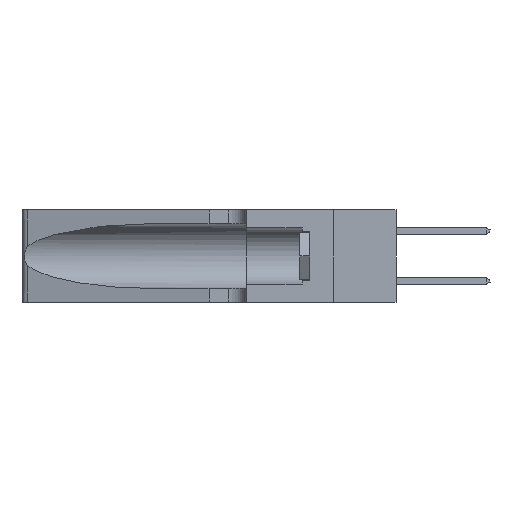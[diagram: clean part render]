
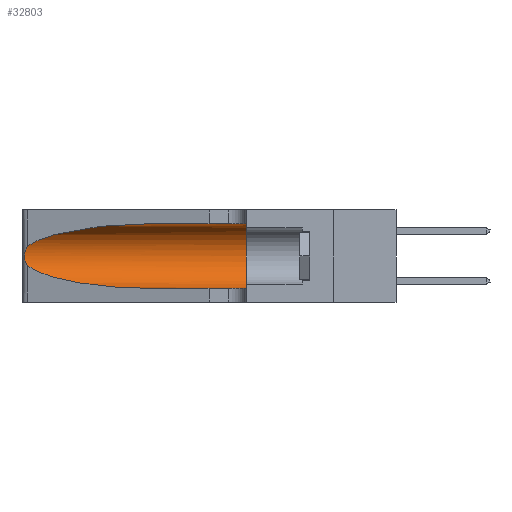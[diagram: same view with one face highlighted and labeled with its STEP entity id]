
A CAD part, left-side view. The second image highlights one B-rep face of the part: STEP entity #32803.
In plain terms, the highlighted cylindrical face has radius 3.308 mm (diameter 6.617 mm), a partial arc.
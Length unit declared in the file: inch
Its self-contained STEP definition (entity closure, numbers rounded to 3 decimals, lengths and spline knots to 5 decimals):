
#409 = VERTEX_POINT ( 'NONE', #32233 ) ;
#2786 = CARTESIAN_POINT ( 'NONE',  ( 0.26017, 1.23833, 0.17102 ) ) ;
#2938 = CARTESIAN_POINT ( 'NONE',  ( 0.25854, 1.2359, 0.20912 ) ) ;
#4188 = AXIS2_PLACEMENT_3D ( 'NONE', #8085, #33717, #25704 ) ;
#4823 = EDGE_CURVE ( 'NONE', #28639, #14928, #31221, .T. ) ;
#6222 = DIRECTION ( 'NONE',  ( 0., -1., 0. ) ) ;
#6497 = ORIENTED_EDGE ( 'NONE', *, *, #22093, .F. ) ;
#6496 = CARTESIAN_POINT ( 'NONE',  ( 0.25789, 1.23486, 0.15765 ) ) ;
#8085 = CARTESIAN_POINT ( 'NONE',  ( 0.1305, 0.35, 0.185 ) ) ;
#8972 = ORIENTED_EDGE ( 'NONE', *, *, #34761, .T. ) ;
#9079 = CARTESIAN_POINT ( 'NONE',  ( 0.1305, 0.35, 0.31525 ) ) ;
#9128 = LINE ( 'NONE', #35742, #40098 ) ;
#10002 = CARTESIAN_POINT ( 'NONE',  ( 0.25487, 1.22718, 0.14631 ) ) ;
#11672 = CARTESIAN_POINT ( 'NONE',  ( 0.18966, 0.96281, 0.31525 ) ) ;
#11804 = DIRECTION ( 'NONE',  ( 0., -1., 0. ) ) ;
#11962 = CARTESIAN_POINT ( 'NONE',  ( 0.1305, 1.61858, 0.185 ) ) ;
#14061 = CARTESIAN_POINT ( 'NONE',  ( 0.26018, 1.23835, 0.19895 ) ) ;
#14373 = CARTESIAN_POINT ( 'NONE',  ( 0.26075, 1.23896, 0.19203 ) ) ;
#14928 = VERTEX_POINT ( 'NONE', #27453 ) ;
#16076 = EDGE_LOOP ( 'NONE', ( #20208, #30236, #8972, #41816, #6497, #32143 ) ) ;
#16143 = VERTEX_POINT ( 'NONE', #9079 ) ;
#17191 = B_SPLINE_CURVE_WITH_KNOTS ( 'NONE', 3,
 ( #43513, #24772, #29067, #46709, #2938, #14061, #14373, #25227, #2786, #21719, #6496, #39848, #32140, #28915 ),
 .UNSPECIFIED., .F., .F.,
 ( 4, 2, 2, 2, 2, 2, 4 ),
 ( 0., 0.00027, 0.00053, 0.00107, 0.0016, 0.00187, 0.00214 ),
 .UNSPECIFIED. ) ;
#17555 = CARTESIAN_POINT ( 'NONE',  ( 0.18966, 0.96281, 0.05475 ) ) ;
#17965 = EDGE_CURVE ( 'NONE', #409, #37661, #17191, .T. ) ;
#18624 =( BOUNDED_CURVE ( )  B_SPLINE_CURVE ( 3, ( #10002, #20283, #17555, #21398 ),
 .UNSPECIFIED., .F., .T. ) 
 B_SPLINE_CURVE_WITH_KNOTS ( ( 4, 4 ),
 ( 3.44316, 4.71239 ),
 .UNSPECIFIED. ) 
 CURVE ( )  GEOMETRIC_REPRESENTATION_ITEM ( )  RATIONAL_B_SPLINE_CURVE ( ( 1., 0.87, 0.87, 1. ) ) 
 REPRESENTATION_ITEM ( '' )  );
#19201 = CARTESIAN_POINT ( 'NONE',  ( 0.1305, 0.72297, 0.31525 ) ) ;
#19380 = EDGE_CURVE ( 'NONE', #37671, #409, #31523, .T. ) ;
#20208 = ORIENTED_EDGE ( 'NONE', *, *, #19380, .T. ) ;
#20212 = CARTESIAN_POINT ( 'NONE',  ( 0.1305, 0.72297, 0.31525 ) ) ;
#20283 = CARTESIAN_POINT ( 'NONE',  ( 0.2373, 1.15595, 0.08982 ) ) ;
#21169 = EDGE_CURVE ( 'NONE', #37671, #16143, #9128, .T. ) ;
#21398 = CARTESIAN_POINT ( 'NONE',  ( 0.1305, 0.72297, 0.05475 ) ) ;
#21719 = CARTESIAN_POINT ( 'NONE',  ( 0.25856, 1.23593, 0.16098 ) ) ;
#22093 = EDGE_CURVE ( 'NONE', #16143, #14928, #23360, .T. ) ;
#23360 = CIRCLE ( 'NONE', #4188, 0.13025 ) ;
#23750 = CARTESIAN_POINT ( 'NONE',  ( 0.25487, 1.22718, 0.14631 ) ) ;
#24772 = CARTESIAN_POINT ( 'NONE',  ( 0.25555, 1.22994, 0.2215 ) ) ;
#25227 = CARTESIAN_POINT ( 'NONE',  ( 0.26075, 1.23896, 0.178 ) ) ;
#25704 = DIRECTION ( 'NONE',  ( 0., 0., 1. ) ) ;
#26779 = DIRECTION ( 'NONE',  ( 0., -1., 0. ) ) ;
#27453 = CARTESIAN_POINT ( 'NONE',  ( 0.1305, 0.35, 0.05475 ) ) ;
#28639 = VERTEX_POINT ( 'NONE', #34189 ) ;
#28915 = CARTESIAN_POINT ( 'NONE',  ( 0.25487, 1.22718, 0.14631 ) ) ;
#29067 = CARTESIAN_POINT ( 'NONE',  ( 0.25639, 1.23184, 0.21858 ) ) ;
#29583 = CARTESIAN_POINT ( 'NONE',  ( 0.2373, 1.15595, 0.28018 ) ) ;
#30045 = VECTOR ( 'NONE', #26779, 39.37008 ) ;
#30065 = CARTESIAN_POINT ( 'NONE',  ( 0.25487, 1.22718, 0.22369 ) ) ;
#30236 = ORIENTED_EDGE ( 'NONE', *, *, #17965, .T. ) ;
#31221 = LINE ( 'NONE', #41539, #30045 ) ;
#31523 =( BOUNDED_CURVE ( )  B_SPLINE_CURVE ( 3, ( #19201, #11672, #29583, #30065 ),
 .UNSPECIFIED., .F., .F. ) 
 B_SPLINE_CURVE_WITH_KNOTS ( ( 4, 4 ),
 ( 1.5708, 2.84003 ),
 .UNSPECIFIED. ) 
 CURVE ( )  GEOMETRIC_REPRESENTATION_ITEM ( )  RATIONAL_B_SPLINE_CURVE ( ( 1., 0.87, 0.87, 1. ) ) 
 REPRESENTATION_ITEM ( '' )  );
#32140 = CARTESIAN_POINT ( 'NONE',  ( 0.25555, 1.22993, 0.14849 ) ) ;
#32143 = ORIENTED_EDGE ( 'NONE', *, *, #21169, .F. ) ;
#32233 = CARTESIAN_POINT ( 'NONE',  ( 0.25487, 1.22718, 0.22369 ) ) ;
#32803 = ADVANCED_FACE ( 'NONE', ( #33558 ), #43322, .F. ) ;
#33558 = FACE_OUTER_BOUND ( 'NONE', #16076, .T. ) ;
#33717 = DIRECTION ( 'NONE',  ( 0., 1., 0. ) ) ;
#34189 = CARTESIAN_POINT ( 'NONE',  ( 0.1305, 0.72297, 0.05475 ) ) ;
#34761 = EDGE_CURVE ( 'NONE', #37661, #28639, #18624, .T. ) ;
#35742 = CARTESIAN_POINT ( 'NONE',  ( 0.1305, 1.61858, 0.31525 ) ) ;
#37469 = DIRECTION ( 'NONE',  ( 0., 0., -1. ) ) ;
#37661 = VERTEX_POINT ( 'NONE', #23750 ) ;
#37671 = VERTEX_POINT ( 'NONE', #20212 ) ;
#39828 = AXIS2_PLACEMENT_3D ( 'NONE', #11962, #11804, #37469 ) ;
#39848 = CARTESIAN_POINT ( 'NONE',  ( 0.25639, 1.23186, 0.15144 ) ) ;
#40098 = VECTOR ( 'NONE', #6222, 39.37008 ) ;
#41539 = CARTESIAN_POINT ( 'NONE',  ( 0.1305, 1.61858, 0.05475 ) ) ;
#41816 = ORIENTED_EDGE ( 'NONE', *, *, #4823, .T. ) ;
#43322 = CYLINDRICAL_SURFACE ( 'NONE', #39828, 0.13025 ) ;
#43513 = CARTESIAN_POINT ( 'NONE',  ( 0.25487, 1.22718, 0.22369 ) ) ;
#46709 = CARTESIAN_POINT ( 'NONE',  ( 0.25787, 1.23484, 0.2124 ) ) ;
